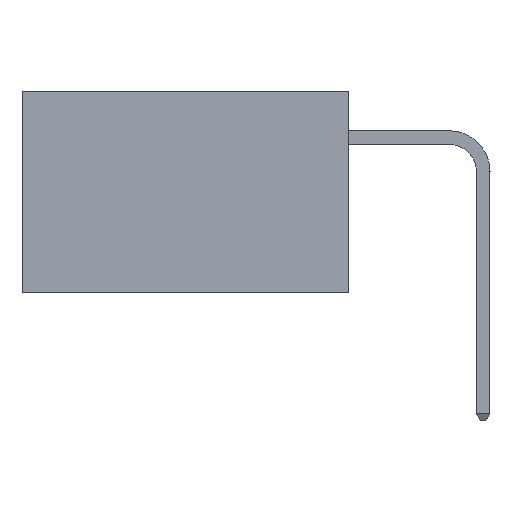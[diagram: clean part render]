
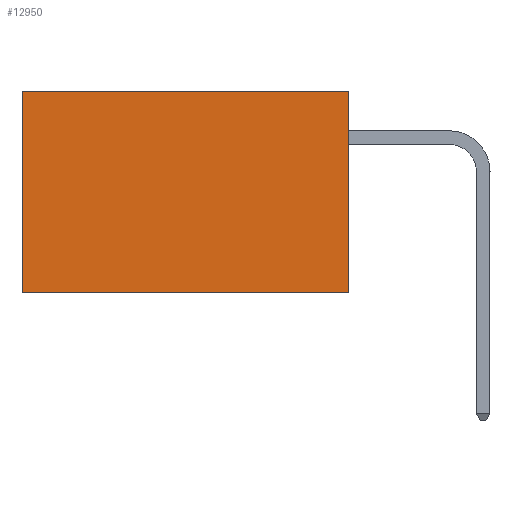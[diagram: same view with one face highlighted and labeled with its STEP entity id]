
A CAD part, left-side view. The second image highlights one B-rep face of the part: STEP entity #12950.
In plain terms, the highlighted planar face has unit normal (-1, 0, 0).
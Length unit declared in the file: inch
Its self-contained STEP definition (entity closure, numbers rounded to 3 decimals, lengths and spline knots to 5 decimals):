
#341 = CARTESIAN_POINT ( 'NONE',  ( 0.2875, 0., 0. ) ) ;
#440 = CARTESIAN_POINT ( 'NONE',  ( 0.2875, 0., -0.37 ) ) ;
#471 = VECTOR ( 'NONE', #16126, 39.37008 ) ;
#755 = ORIENTED_EDGE ( 'NONE', *, *, #7468, .F. ) ;
#1130 = VERTEX_POINT ( 'NONE', #9186 ) ;
#1966 = CARTESIAN_POINT ( 'NONE',  ( 0.2875, 0., 0. ) ) ;
#2881 = ORIENTED_EDGE ( 'NONE', *, *, #6215, .T. ) ;
#5968 = DIRECTION ( 'NONE',  ( 0., 1., 0. ) ) ;
#6215 = EDGE_CURVE ( 'NONE', #10527, #11902, #10784, .T. ) ;
#6694 = PLANE ( 'NONE',  #12287 ) ;
#7262 = VECTOR ( 'NONE', #11063, 39.37008 ) ;
#7468 = EDGE_CURVE ( 'NONE', #1130, #10720, #8061, .T. ) ;
#7986 = DIRECTION ( 'NONE',  ( 0., 0., -1. ) ) ;
#8061 = LINE ( 'NONE', #341, #7262 ) ;
#8609 = VECTOR ( 'NONE', #5968, 39.37008 ) ;
#9186 = CARTESIAN_POINT ( 'NONE',  ( 0.2875, 0., 0. ) ) ;
#9224 = EDGE_LOOP ( 'NONE', ( #2881, #13040, #755, #16956 ) ) ;
#9234 = LINE ( 'NONE', #1966, #12342 ) ;
#10170 = CARTESIAN_POINT ( 'NONE',  ( 0.2875, 0.6, 0. ) ) ;
#10473 = FACE_OUTER_BOUND ( 'NONE', #9224, .T. ) ;
#10527 = VERTEX_POINT ( 'NONE', #15442 ) ;
#10720 = VERTEX_POINT ( 'NONE', #17088 ) ;
#10784 = LINE ( 'NONE', #10170, #471 ) ;
#11063 = DIRECTION ( 'NONE',  ( 0., 0., -1. ) ) ;
#11335 = DIRECTION ( 'NONE',  ( 0., 1., 0. ) ) ;
#11902 = VERTEX_POINT ( 'NONE', #16896 ) ;
#11919 = CARTESIAN_POINT ( 'NONE',  ( 0.2875, 0., 0. ) ) ;
#12287 = AXIS2_PLACEMENT_3D ( 'NONE', #11919, #15816, #7986 ) ;
#12342 = VECTOR ( 'NONE', #11335, 39.37008 ) ;
#12950 = ADVANCED_FACE ( 'NONE', ( #10473 ), #6694, .F. ) ;
#12986 = LINE ( 'NONE', #440, #8609 ) ;
#13040 = ORIENTED_EDGE ( 'NONE', *, *, #13240, .F. ) ;
#13240 = EDGE_CURVE ( 'NONE', #10720, #11902, #12986, .T. ) ;
#15442 = CARTESIAN_POINT ( 'NONE',  ( 0.2875, 0.6, 0. ) ) ;
#15816 = DIRECTION ( 'NONE',  ( 1., 0., 0. ) ) ;
#16126 = DIRECTION ( 'NONE',  ( 0., 0., -1. ) ) ;
#16698 = EDGE_CURVE ( 'NONE', #1130, #10527, #9234, .T. ) ;
#16896 = CARTESIAN_POINT ( 'NONE',  ( 0.2875, 0.6, -0.37 ) ) ;
#16956 = ORIENTED_EDGE ( 'NONE', *, *, #16698, .T. ) ;
#17088 = CARTESIAN_POINT ( 'NONE',  ( 0.2875, 0., -0.37 ) ) ;
